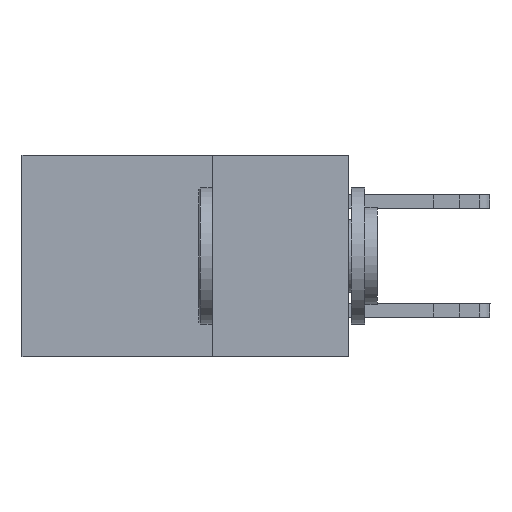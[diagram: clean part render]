
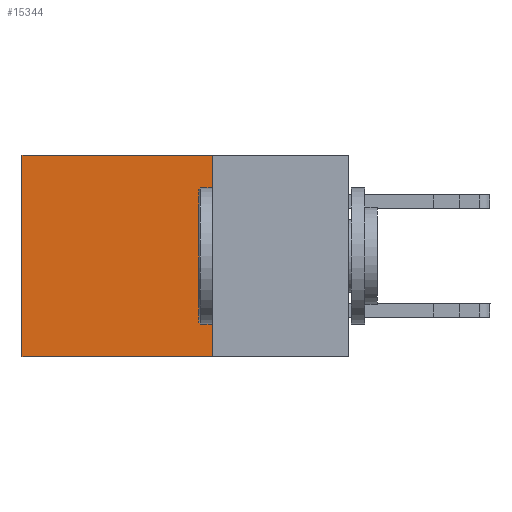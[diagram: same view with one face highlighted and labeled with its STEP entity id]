
A CAD part, left-side view. The second image highlights one B-rep face of the part: STEP entity #15344.
In plain terms, the highlighted planar face has unit normal (-1, 0, 0).
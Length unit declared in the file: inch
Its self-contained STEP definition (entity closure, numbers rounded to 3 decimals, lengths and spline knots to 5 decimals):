
#356 = ORIENTED_EDGE ( 'NONE', *, *, #6513, .F. ) ;
#443 = VECTOR ( 'NONE', #7913, 39.37008 ) ;
#830 = LINE ( 'NONE', #8263, #443 ) ;
#1139 = LINE ( 'NONE', #9953, #3632 ) ;
#1325 = LINE ( 'NONE', #6868, #4072 ) ;
#1480 = EDGE_LOOP ( 'NONE', ( #5115, #356, #14058, #5918 ) ) ;
#1770 = EDGE_CURVE ( 'NONE', #14392, #4883, #1325, .T. ) ;
#2145 = DIRECTION ( 'NONE',  ( 0., 1., 0. ) ) ;
#2581 = EDGE_CURVE ( 'NONE', #14392, #12884, #1139, .T. ) ;
#3632 = VECTOR ( 'NONE', #7932, 39.37008 ) ;
#4072 = VECTOR ( 'NONE', #2145, 39.37008 ) ;
#4883 = VERTEX_POINT ( 'NONE', #10535 ) ;
#5115 = ORIENTED_EDGE ( 'NONE', *, *, #8563, .T. ) ;
#5336 = CARTESIAN_POINT ( 'NONE',  ( 0.2615, 0.25, 0. ) ) ;
#5918 = ORIENTED_EDGE ( 'NONE', *, *, #1770, .T. ) ;
#6513 = EDGE_CURVE ( 'NONE', #12884, #12782, #830, .T. ) ;
#6868 = CARTESIAN_POINT ( 'NONE',  ( 0.2615, 0.25, 0. ) ) ;
#7913 = DIRECTION ( 'NONE',  ( 0., 1., 0. ) ) ;
#7932 = DIRECTION ( 'NONE',  ( 0., 0., -1. ) ) ;
#8240 = VECTOR ( 'NONE', #12728, 39.37008 ) ;
#8263 = CARTESIAN_POINT ( 'NONE',  ( 0.2615, 0.25, -0.37 ) ) ;
#8407 = DIRECTION ( 'NONE',  ( 0., 0., -1. ) ) ;
#8563 = EDGE_CURVE ( 'NONE', #4883, #12782, #14408, .T. ) ;
#9953 = CARTESIAN_POINT ( 'NONE',  ( 0.2615, 0.25, -0.37 ) ) ;
#10535 = CARTESIAN_POINT ( 'NONE',  ( 0.2615, 0.6, 0. ) ) ;
#11004 = PLANE ( 'NONE',  #15574 ) ;
#11600 = CARTESIAN_POINT ( 'NONE',  ( 0.2615, 0.6, -0.37 ) ) ;
#12153 = CARTESIAN_POINT ( 'NONE',  ( 0.2615, 0.25, -0.37 ) ) ;
#12479 = CARTESIAN_POINT ( 'NONE',  ( 0.2615, 0.6, -0.37 ) ) ;
#12728 = DIRECTION ( 'NONE',  ( 0., 0., -1. ) ) ;
#12782 = VERTEX_POINT ( 'NONE', #11600 ) ;
#12884 = VERTEX_POINT ( 'NONE', #14106 ) ;
#14058 = ORIENTED_EDGE ( 'NONE', *, *, #2581, .F. ) ;
#14106 = CARTESIAN_POINT ( 'NONE',  ( 0.2615, 0.25, -0.37 ) ) ;
#14392 = VERTEX_POINT ( 'NONE', #5336 ) ;
#14408 = LINE ( 'NONE', #12479, #8240 ) ;
#14442 = FACE_OUTER_BOUND ( 'NONE', #1480, .T. ) ;
#15344 = ADVANCED_FACE ( 'NONE', ( #14442 ), #11004, .F. ) ;
#15574 = AXIS2_PLACEMENT_3D ( 'NONE', #12153, #15630, #8407 ) ;
#15630 = DIRECTION ( 'NONE',  ( 1., 0., 0. ) ) ;
